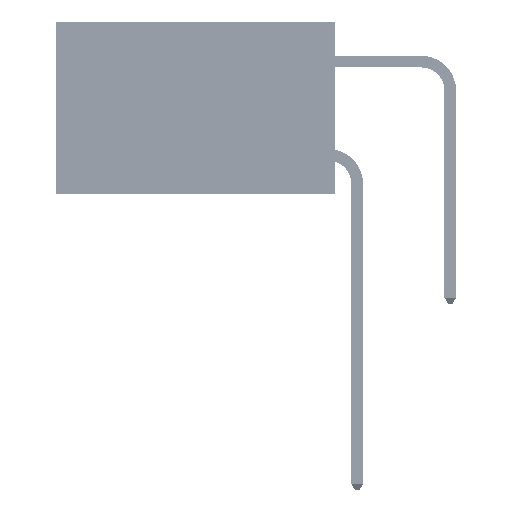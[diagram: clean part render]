
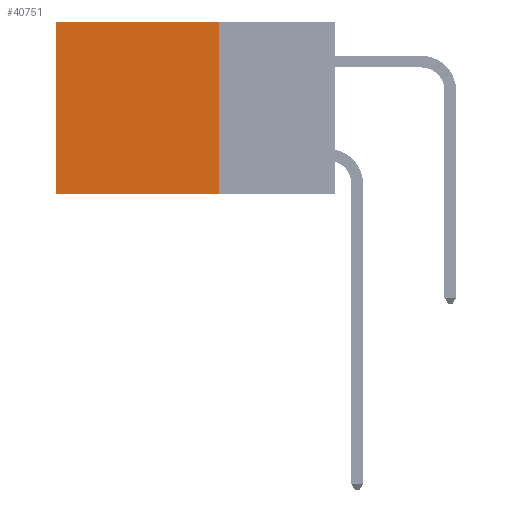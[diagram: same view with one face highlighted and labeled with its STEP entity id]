
A CAD part, left-side view. The second image highlights one B-rep face of the part: STEP entity #40751.
In plain terms, the highlighted planar face has unit normal (-1, 0, 0).
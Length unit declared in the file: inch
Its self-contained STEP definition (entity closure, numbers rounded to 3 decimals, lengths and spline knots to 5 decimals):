
#19 = VECTOR ( 'NONE', #1560, 39.37008 ) ;
#1160 = ORIENTED_EDGE ( 'NONE', *, *, #6473, .T. ) ;
#1560 = DIRECTION ( 'NONE',  ( 0., 0., -1. ) ) ;
#1939 = LINE ( 'NONE', #39635, #26749 ) ;
#4509 = DIRECTION ( 'NONE',  ( 1., 0., 0. ) ) ;
#4846 = EDGE_CURVE ( 'NONE', #44429, #19009, #19118, .T. ) ;
#6447 = ORIENTED_EDGE ( 'NONE', *, *, #32265, .F. ) ;
#6473 = EDGE_CURVE ( 'NONE', #19009, #6677, #21957, .T. ) ;
#6677 = VERTEX_POINT ( 'NONE', #11410 ) ;
#9069 = DIRECTION ( 'NONE',  ( 0., 0., -1. ) ) ;
#9223 = DIRECTION ( 'NONE',  ( 0., 1., 0. ) ) ;
#10382 = AXIS2_PLACEMENT_3D ( 'NONE', #27147, #4509, #19722 ) ;
#11410 = CARTESIAN_POINT ( 'NONE',  ( 0.2875, 0.6, -0.37 ) ) ;
#14161 = CARTESIAN_POINT ( 'NONE',  ( 0.2875, 0.25, 0. ) ) ;
#15982 = CARTESIAN_POINT ( 'NONE',  ( 0.2875, 0.25, -0.37 ) ) ;
#16026 = FACE_OUTER_BOUND ( 'NONE', #36740, .T. ) ;
#19009 = VERTEX_POINT ( 'NONE', #38837 ) ;
#19118 = LINE ( 'NONE', #27540, #41006 ) ;
#19722 = DIRECTION ( 'NONE',  ( 0., 0., -1. ) ) ;
#20944 = CARTESIAN_POINT ( 'NONE',  ( 0.2875, 0.6, 0. ) ) ;
#21922 = ORIENTED_EDGE ( 'NONE', *, *, #26904, .F. ) ;
#21957 = LINE ( 'NONE', #20944, #45611 ) ;
#26749 = VECTOR ( 'NONE', #42920, 39.37008 ) ;
#26904 = EDGE_CURVE ( 'NONE', #44429, #38541, #42626, .T. ) ;
#27147 = CARTESIAN_POINT ( 'NONE',  ( 0.2875, 0.25, 0. ) ) ;
#27540 = CARTESIAN_POINT ( 'NONE',  ( 0.2875, 0.25, 0. ) ) ;
#29987 = ORIENTED_EDGE ( 'NONE', *, *, #4846, .T. ) ;
#32265 = EDGE_CURVE ( 'NONE', #38541, #6677, #1939, .T. ) ;
#36740 = EDGE_LOOP ( 'NONE', ( #1160, #6447, #21922, #29987 ) ) ;
#38541 = VERTEX_POINT ( 'NONE', #15982 ) ;
#38837 = CARTESIAN_POINT ( 'NONE',  ( 0.2875, 0.6, 0. ) ) ;
#39272 = CARTESIAN_POINT ( 'NONE',  ( 0.2875, 0.25, 0. ) ) ;
#39635 = CARTESIAN_POINT ( 'NONE',  ( 0.2875, 0.25, -0.37 ) ) ;
#40751 = ADVANCED_FACE ( 'NONE', ( #16026 ), #45829, .F. ) ;
#41006 = VECTOR ( 'NONE', #9223, 39.37008 ) ;
#42626 = LINE ( 'NONE', #39272, #19 ) ;
#42920 = DIRECTION ( 'NONE',  ( 0., 1., 0. ) ) ;
#44429 = VERTEX_POINT ( 'NONE', #14161 ) ;
#45611 = VECTOR ( 'NONE', #9069, 39.37008 ) ;
#45829 = PLANE ( 'NONE',  #10382 ) ;
